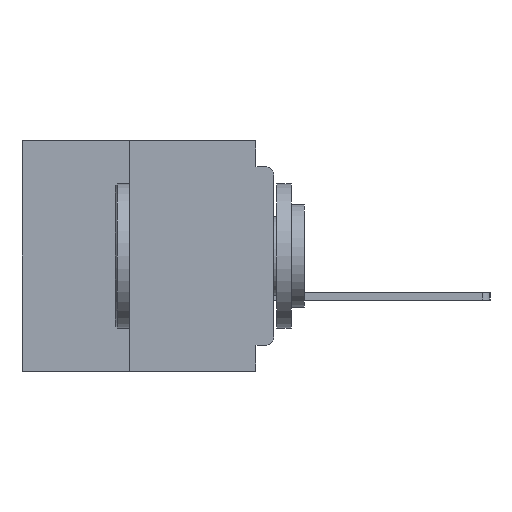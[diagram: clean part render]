
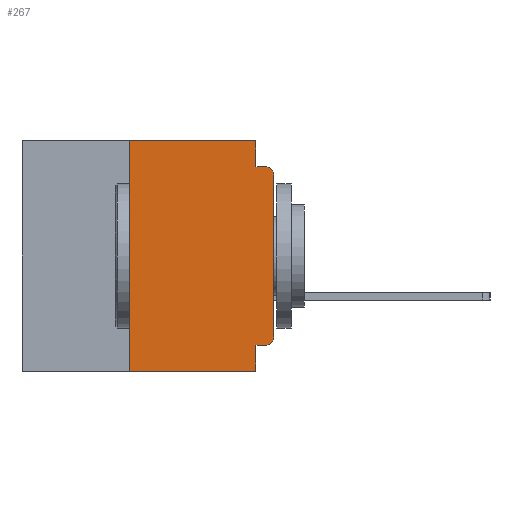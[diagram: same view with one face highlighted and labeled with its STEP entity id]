
A CAD part, left-side view. The second image highlights one B-rep face of the part: STEP entity #267.
In plain terms, the highlighted planar face has unit normal (-1, 0, 0).
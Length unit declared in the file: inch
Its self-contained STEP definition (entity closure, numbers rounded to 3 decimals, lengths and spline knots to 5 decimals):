
#267 = ADVANCED_FACE ( 'NONE', ( #26462 ), #9780, .F. ) ;
#305 = ORIENTED_EDGE ( 'NONE', *, *, #2326, .T. ) ;
#1053 = VERTEX_POINT ( 'NONE', #19269 ) ;
#2326 = EDGE_CURVE ( 'NONE', #36159, #23972, #12451, .T. ) ;
#2745 = DIRECTION ( 'NONE',  ( 0., -1., 0. ) ) ;
#3205 = ORIENTED_EDGE ( 'NONE', *, *, #4429, .F. ) ;
#3393 = VERTEX_POINT ( 'NONE', #4142 ) ;
#3417 = CARTESIAN_POINT ( 'NONE',  ( 0., 0.015, -0.06 ) ) ;
#4142 = CARTESIAN_POINT ( 'NONE',  ( 0., 0.031, -0.4 ) ) ;
#4318 = VERTEX_POINT ( 'NONE', #44858 ) ;
#4429 = EDGE_CURVE ( 'NONE', #36159, #28112, #16331, .T. ) ;
#4439 = AXIS2_PLACEMENT_3D ( 'NONE', #25667, #12606, #14126 ) ;
#4510 = VERTEX_POINT ( 'NONE', #40079 ) ;
#5011 = EDGE_CURVE ( 'NONE', #28112, #3393, #10525, .T. ) ;
#5093 = AXIS2_PLACEMENT_3D ( 'NONE', #3417, #29222, #7172 ) ;
#5398 = CARTESIAN_POINT ( 'NONE',  ( 0., 0.25, 0. ) ) ;
#6030 = VECTOR ( 'NONE', #12649, 39.37008 ) ;
#6045 = ORIENTED_EDGE ( 'NONE', *, *, #41217, .T. ) ;
#6095 = LINE ( 'NONE', #18513, #24519 ) ;
#6305 = LINE ( 'NONE', #24203, #32195 ) ;
#6744 = CIRCLE ( 'NONE', #5093, 0.015 ) ;
#7172 = DIRECTION ( 'NONE',  ( 0., 0., -1. ) ) ;
#8281 = CARTESIAN_POINT ( 'NONE',  ( 0., 0., -0.06 ) ) ;
#8779 = ORIENTED_EDGE ( 'NONE', *, *, #12229, .F. ) ;
#9526 = CARTESIAN_POINT ( 'NONE',  ( 0., 0.031, 0. ) ) ;
#9780 = PLANE ( 'NONE',  #4439 ) ;
#9945 = ORIENTED_EDGE ( 'NONE', *, *, #5011, .F. ) ;
#10429 = VECTOR ( 'NONE', #2745, 39.37008 ) ;
#10525 = LINE ( 'NONE', #27842, #20235 ) ;
#12229 = EDGE_CURVE ( 'NONE', #44634, #4510, #6305, .T. ) ;
#12451 = CIRCLE ( 'NONE', #21806, 0.015 ) ;
#12606 = DIRECTION ( 'NONE',  ( 1., 0., 0. ) ) ;
#12628 = VERTEX_POINT ( 'NONE', #8281 ) ;
#12649 = DIRECTION ( 'NONE',  ( 0., -1., 0. ) ) ;
#13496 = CARTESIAN_POINT ( 'NONE',  ( 0., 0., -0.34 ) ) ;
#14007 = VECTOR ( 'NONE', #42867, 39.37008 ) ;
#14126 = DIRECTION ( 'NONE',  ( 0., 0., -1. ) ) ;
#16331 = LINE ( 'NONE', #42240, #34641 ) ;
#17409 = CARTESIAN_POINT ( 'NONE',  ( 0., 0.437, -0.4 ) ) ;
#17617 = EDGE_CURVE ( 'NONE', #37228, #44634, #34197, .T. ) ;
#18513 = CARTESIAN_POINT ( 'NONE',  ( 0., 0.25, -0.4 ) ) ;
#19269 = CARTESIAN_POINT ( 'NONE',  ( 0., 0.25, -0.4 ) ) ;
#20174 = ORIENTED_EDGE ( 'NONE', *, *, #17617, .F. ) ;
#20235 = VECTOR ( 'NONE', #27990, 39.37008 ) ;
#21092 = CARTESIAN_POINT ( 'NONE',  ( 0., 0.015, -0.355 ) ) ;
#21244 = VECTOR ( 'NONE', #27844, 39.37008 ) ;
#21806 = AXIS2_PLACEMENT_3D ( 'NONE', #37059, #36968, #36867 ) ;
#22404 = LINE ( 'NONE', #24142, #21244 ) ;
#23733 = LINE ( 'NONE', #17409, #14007 ) ;
#23972 = VERTEX_POINT ( 'NONE', #13496 ) ;
#24142 = CARTESIAN_POINT ( 'NONE',  ( 0., 0., 0. ) ) ;
#24203 = CARTESIAN_POINT ( 'NONE',  ( 0., 0.031, 0. ) ) ;
#24519 = VECTOR ( 'NONE', #44873, 39.37008 ) ;
#25667 = CARTESIAN_POINT ( 'NONE',  ( 0., 0.437, 0. ) ) ;
#25674 = ORIENTED_EDGE ( 'NONE', *, *, #33752, .F. ) ;
#26462 = FACE_OUTER_BOUND ( 'NONE', #43309, .T. ) ;
#27466 = EDGE_CURVE ( 'NONE', #1053, #3393, #23733, .T. ) ;
#27842 = CARTESIAN_POINT ( 'NONE',  ( 0., 0.031, -0.4 ) ) ;
#27844 = DIRECTION ( 'NONE',  ( 0., 0., 1. ) ) ;
#27990 = DIRECTION ( 'NONE',  ( 0., 0., -1. ) ) ;
#28112 = VERTEX_POINT ( 'NONE', #28217 ) ;
#28217 = CARTESIAN_POINT ( 'NONE',  ( 0., 0.031, -0.355 ) ) ;
#28538 = CARTESIAN_POINT ( 'NONE',  ( 0., 0., -0.045 ) ) ;
#29222 = DIRECTION ( 'NONE',  ( -1., 0., 0. ) ) ;
#30934 = CARTESIAN_POINT ( 'NONE',  ( 0., 0.437, 0. ) ) ;
#32195 = VECTOR ( 'NONE', #35228, 39.37008 ) ;
#33752 = EDGE_CURVE ( 'NONE', #4510, #4318, #46833, .T. ) ;
#34197 = LINE ( 'NONE', #30934, #6030 ) ;
#34641 = VECTOR ( 'NONE', #42304, 39.37008 ) ;
#35228 = DIRECTION ( 'NONE',  ( 0., 0., -1. ) ) ;
#36159 = VERTEX_POINT ( 'NONE', #21092 ) ;
#36867 = DIRECTION ( 'NONE',  ( 0., 0., -1. ) ) ;
#36968 = DIRECTION ( 'NONE',  ( -1., 0., 0. ) ) ;
#37059 = CARTESIAN_POINT ( 'NONE',  ( 0., 0.015, -0.34 ) ) ;
#37228 = VERTEX_POINT ( 'NONE', #5398 ) ;
#37937 = ORIENTED_EDGE ( 'NONE', *, *, #27466, .T. ) ;
#39800 = EDGE_CURVE ( 'NONE', #1053, #37228, #6095, .T. ) ;
#40079 = CARTESIAN_POINT ( 'NONE',  ( 0., 0.031, -0.045 ) ) ;
#41217 = EDGE_CURVE ( 'NONE', #23972, #12628, #22404, .T. ) ;
#42240 = CARTESIAN_POINT ( 'NONE',  ( 0., 0., -0.355 ) ) ;
#42304 = DIRECTION ( 'NONE',  ( 0., 1., 0. ) ) ;
#42867 = DIRECTION ( 'NONE',  ( 0., -1., 0. ) ) ;
#43244 = EDGE_CURVE ( 'NONE', #12628, #4318, #6744, .T. ) ;
#43309 = EDGE_LOOP ( 'NONE', ( #6045, #44344, #25674, #8779, #20174, #46325, #37937, #9945, #3205, #305 ) ) ;
#44344 = ORIENTED_EDGE ( 'NONE', *, *, #43244, .T. ) ;
#44634 = VERTEX_POINT ( 'NONE', #9526 ) ;
#44858 = CARTESIAN_POINT ( 'NONE',  ( 0., 0.015, -0.045 ) ) ;
#44873 = DIRECTION ( 'NONE',  ( 0., 0., 1. ) ) ;
#46325 = ORIENTED_EDGE ( 'NONE', *, *, #39800, .F. ) ;
#46833 = LINE ( 'NONE', #28538, #10429 ) ;
